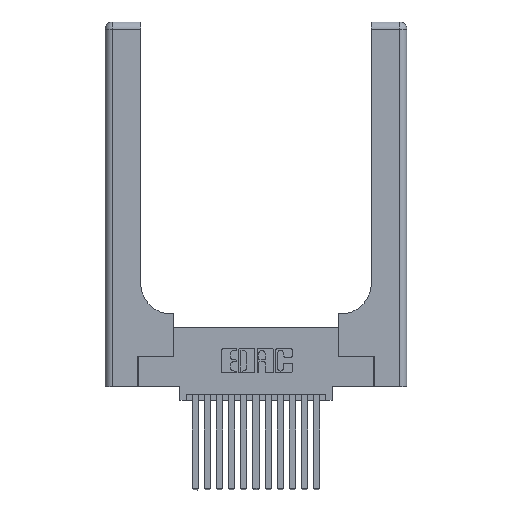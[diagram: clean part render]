
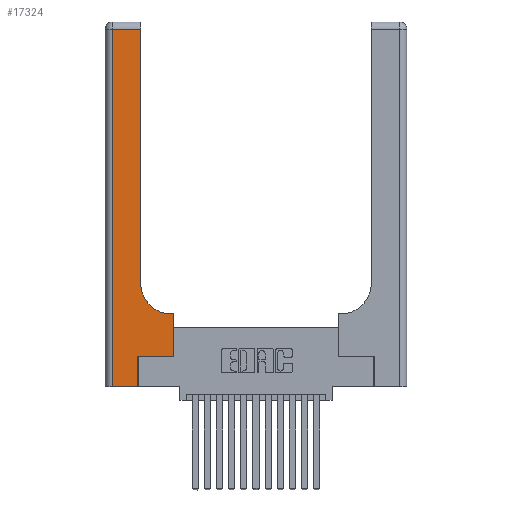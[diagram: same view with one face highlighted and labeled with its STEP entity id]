
A CAD part, top view. The second image highlights one B-rep face of the part: STEP entity #17324.
In plain terms, the highlighted planar face has unit normal (0, 0, 1).
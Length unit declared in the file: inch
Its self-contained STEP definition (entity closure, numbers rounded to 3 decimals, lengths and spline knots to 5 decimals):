
#113 = DIRECTION ( 'NONE',  ( 0., 1., 0. ) ) ;
#226 = VECTOR ( 'NONE', #16546, 39.37008 ) ;
#571 = CARTESIAN_POINT ( 'NONE',  ( 0.269, 0.25, 0.37 ) ) ;
#683 = EDGE_CURVE ( 'NONE', #10729, #13208, #6269, .T. ) ;
#705 = CARTESIAN_POINT ( 'NONE',  ( 0.5585, 0.25, 0.37 ) ) ;
#861 = VECTOR ( 'NONE', #13547, 39.37008 ) ;
#1152 = CARTESIAN_POINT ( 'NONE',  ( 0., 0., 0.37 ) ) ;
#1209 = VECTOR ( 'NONE', #113, 39.37008 ) ;
#1292 = CARTESIAN_POINT ( 'NONE',  ( 0.06, 3., 0.37 ) ) ;
#1352 = CARTESIAN_POINT ( 'NONE',  ( 0., 3., 0.37 ) ) ;
#1611 = EDGE_CURVE ( 'NONE', #3001, #3583, #5387, .T. ) ;
#1700 = CARTESIAN_POINT ( 'NONE',  ( 0.5415, 0.6, 0.37 ) ) ;
#1822 = AXIS2_PLACEMENT_3D ( 'NONE', #1352, #14957, #10861 ) ;
#1919 = CARTESIAN_POINT ( 'NONE',  ( 0.5415, 0.85, 0.37 ) ) ;
#2344 = DIRECTION ( 'NONE',  ( -1., 0., 0. ) ) ;
#2660 = EDGE_CURVE ( 'NONE', #13208, #10745, #8098, .T. ) ;
#2826 = EDGE_CURVE ( 'NONE', #9807, #10729, #11564, .T. ) ;
#3001 = VERTEX_POINT ( 'NONE', #4503 ) ;
#3583 = VERTEX_POINT ( 'NONE', #16848 ) ;
#4263 = CIRCLE ( 'NONE', #12691, 0.25 ) ;
#4501 = LINE ( 'NONE', #1152, #861 ) ;
#4503 = CARTESIAN_POINT ( 'NONE',  ( 0.2915, 2.94, 0.37 ) ) ;
#4785 = CARTESIAN_POINT ( 'NONE',  ( 0.2915, 0.85, 0.37 ) ) ;
#5036 = VECTOR ( 'NONE', #6146, 39.37008 ) ;
#5387 = LINE ( 'NONE', #9247, #7144 ) ;
#5671 = CARTESIAN_POINT ( 'NONE',  ( 0.269, 0., 0.37 ) ) ;
#6096 = DIRECTION ( 'NONE',  ( 0., 0., -1. ) ) ;
#6146 = DIRECTION ( 'NONE',  ( 0., 1., 0. ) ) ;
#6236 = ORIENTED_EDGE ( 'NONE', *, *, #11174, .T. ) ;
#6269 = LINE ( 'NONE', #571, #16266 ) ;
#6301 = FACE_OUTER_BOUND ( 'NONE', #16134, .T. ) ;
#6305 = CARTESIAN_POINT ( 'NONE',  ( 0.269, 0., 0.37 ) ) ;
#6560 = CARTESIAN_POINT ( 'NONE',  ( 0.269, 0.25, 0.37 ) ) ;
#6581 = VERTEX_POINT ( 'NONE', #1700 ) ;
#6625 = ORIENTED_EDGE ( 'NONE', *, *, #14071, .T. ) ;
#7144 = VECTOR ( 'NONE', #2344, 39.37008 ) ;
#8063 = CARTESIAN_POINT ( 'NONE',  ( 0.2915, 0.6, 0.37 ) ) ;
#8098 = LINE ( 'NONE', #705, #5036 ) ;
#8532 = ORIENTED_EDGE ( 'NONE', *, *, #11613, .T. ) ;
#8702 = VERTEX_POINT ( 'NONE', #4785 ) ;
#9124 = CARTESIAN_POINT ( 'NONE',  ( 0.5585, 0.25, 0.37 ) ) ;
#9171 = ORIENTED_EDGE ( 'NONE', *, *, #2660, .T. ) ;
#9247 = CARTESIAN_POINT ( 'NONE',  ( 0., 2.94, 0.37 ) ) ;
#9400 = LINE ( 'NONE', #1292, #14585 ) ;
#9807 = VERTEX_POINT ( 'NONE', #5671 ) ;
#10248 = VECTOR ( 'NONE', #11999, 39.37008 ) ;
#10650 = ORIENTED_EDGE ( 'NONE', *, *, #683, .T. ) ;
#10729 = VERTEX_POINT ( 'NONE', #6560 ) ;
#10730 = CARTESIAN_POINT ( 'NONE',  ( 0.5585, 0.6, 0.37 ) ) ;
#10745 = VERTEX_POINT ( 'NONE', #10730 ) ;
#10786 = PLANE ( 'NONE',  #1822 ) ;
#10861 = DIRECTION ( 'NONE',  ( -1., 0., 0. ) ) ;
#10955 = LINE ( 'NONE', #12443, #1209 ) ;
#11174 = EDGE_CURVE ( 'NONE', #17947, #9807, #4501, .T. ) ;
#11564 = LINE ( 'NONE', #6305, #10248 ) ;
#11611 = DIRECTION ( 'NONE',  ( 1., 0., 0. ) ) ;
#11613 = EDGE_CURVE ( 'NONE', #6581, #8702, #4263, .T. ) ;
#11663 = DIRECTION ( 'NONE',  ( 1., 0., 0. ) ) ;
#11952 = ORIENTED_EDGE ( 'NONE', *, *, #17268, .T. ) ;
#11999 = DIRECTION ( 'NONE',  ( 0., 1., 0. ) ) ;
#12443 = CARTESIAN_POINT ( 'NONE',  ( 0.2915, 3., 0.37 ) ) ;
#12691 = AXIS2_PLACEMENT_3D ( 'NONE', #1919, #6096, #11611 ) ;
#12961 = EDGE_CURVE ( 'NONE', #8702, #3001, #10955, .T. ) ;
#13208 = VERTEX_POINT ( 'NONE', #9124 ) ;
#13547 = DIRECTION ( 'NONE',  ( 1., 0., 0. ) ) ;
#14071 = EDGE_CURVE ( 'NONE', #3583, #17947, #9400, .T. ) ;
#14405 = ORIENTED_EDGE ( 'NONE', *, *, #2826, .T. ) ;
#14585 = VECTOR ( 'NONE', #17845, 39.37008 ) ;
#14942 = ORIENTED_EDGE ( 'NONE', *, *, #12961, .T. ) ;
#14957 = DIRECTION ( 'NONE',  ( 0., 0., -1. ) ) ;
#16134 = EDGE_LOOP ( 'NONE', ( #14942, #17152, #6625, #6236, #14405, #10650, #9171, #11952, #8532 ) ) ;
#16266 = VECTOR ( 'NONE', #11663, 39.37008 ) ;
#16272 = LINE ( 'NONE', #8063, #226 ) ;
#16546 = DIRECTION ( 'NONE',  ( -1., 0., 0. ) ) ;
#16848 = CARTESIAN_POINT ( 'NONE',  ( 0.06, 2.94, 0.37 ) ) ;
#17152 = ORIENTED_EDGE ( 'NONE', *, *, #1611, .T. ) ;
#17268 = EDGE_CURVE ( 'NONE', #10745, #6581, #16272, .T. ) ;
#17324 = ADVANCED_FACE ( 'NONE', ( #6301 ), #10786, .F. ) ;
#17821 = CARTESIAN_POINT ( 'NONE',  ( 0.06, 0., 0.37 ) ) ;
#17845 = DIRECTION ( 'NONE',  ( 0., -1., 0. ) ) ;
#17947 = VERTEX_POINT ( 'NONE', #17821 ) ;
